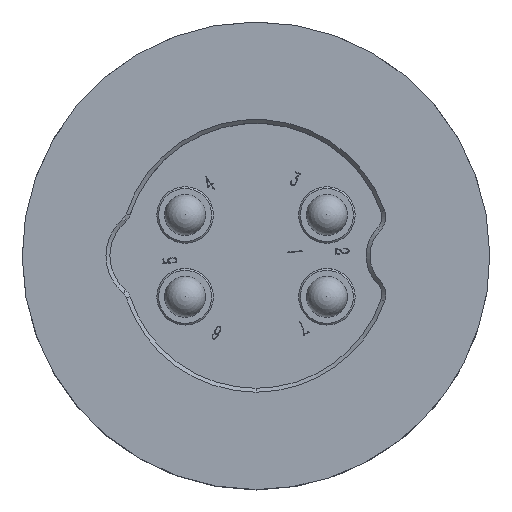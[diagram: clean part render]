
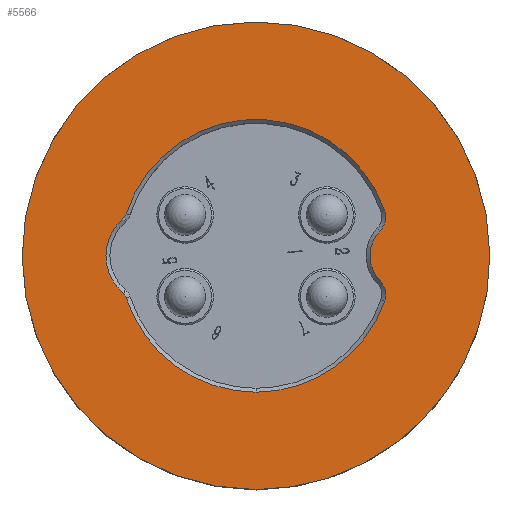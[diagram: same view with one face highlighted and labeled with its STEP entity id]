
A CAD part, top view. The second image highlights one B-rep face of the part: STEP entity #5566.
In plain terms, the highlighted planar face has unit normal (0, 0, 1).
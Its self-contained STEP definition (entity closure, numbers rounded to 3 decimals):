
#47 = DIRECTION ( 'NONE',  ( -1., 0., 0. ) ) ;
#152 = CARTESIAN_POINT ( 'NONE',  ( 0., 0., 0. ) ) ;
#515 = AXIS2_PLACEMENT_3D ( 'NONE', #9456, #1207, #4871 ) ;
#540 = EDGE_CURVE ( 'NONE', #8678, #10685, #4382, .T. ) ;
#756 = CARTESIAN_POINT ( 'NONE',  ( 0., -3.5, 0. ) ) ;
#1207 = DIRECTION ( 'NONE',  ( 0., 0., 1. ) ) ;
#1212 = CARTESIAN_POINT ( 'NONE',  ( 0., 0., 0. ) ) ;
#1215 = DIRECTION ( 'NONE',  ( 0., 0., 1. ) ) ;
#1306 = DIRECTION ( 'NONE',  ( 0.943, -0.332, 0. ) ) ;
#1320 = CARTESIAN_POINT ( 'NONE',  ( -2.6, 0., 0. ) ) ;
#1339 = AXIS2_PLACEMENT_3D ( 'NONE', #9462, #1215, #4879 ) ;
#1507 = EDGE_CURVE ( 'NONE', #4298, #8516, #7248, .T. ) ;
#1793 = ORIENTED_EDGE ( 'NONE', *, *, #2219, .T. ) ;
#1893 = AXIS2_PLACEMENT_3D ( 'NONE', #1320, #4993, #8657 ) ;
#1932 = ORIENTED_EDGE ( 'NONE', *, *, #11006, .T. ) ;
#2031 = CARTESIAN_POINT ( 'NONE',  ( -3.33, -1.079, 0. ) ) ;
#2101 = EDGE_CURVE ( 'NONE', #4407, #4084, #5161, .T. ) ;
#2219 = EDGE_CURVE ( 'NONE', #4084, #4665, #7648, .T. ) ;
#2424 = DIRECTION ( 'NONE',  ( 0.943, -0.332, 0. ) ) ;
#2466 = AXIS2_PLACEMENT_3D ( 'NONE', #11554, #3294, #6956 ) ;
#2517 = DIRECTION ( 'NONE',  ( 0., -1., 0. ) ) ;
#2592 = DIRECTION ( 'NONE',  ( 0.716, 0.698, 0. ) ) ;
#2992 = EDGE_LOOP ( 'NONE', ( #5444, #9931, #11263 ) ) ;
#3232 = VERTEX_POINT ( 'NONE', #7634 ) ;
#3294 = DIRECTION ( 'NONE',  ( 0., 0., -1. ) ) ;
#3421 = AXIS2_PLACEMENT_3D ( 'NONE', #4634, #8295, #47 ) ;
#3426 = PLANE ( 'NONE',  #9767 ) ;
#3532 = DIRECTION ( 'NONE',  ( 0., 0., 1. ) ) ;
#3622 = AXIS2_PLACEMENT_3D ( 'NONE', #11799, #3532, #7199 ) ;
#3653 = CIRCLE ( 'NONE', #10380, 0.5 ) ;
#3708 = CARTESIAN_POINT ( 'NONE',  ( 0., 0., 0. ) ) ;
#3765 = ORIENTED_EDGE ( 'NONE', *, *, #540, .T. ) ;
#3799 = ORIENTED_EDGE ( 'NONE', *, *, #1507, .T. ) ;
#3841 = DIRECTION ( 'NONE',  ( 0., 0., -1. ) ) ;
#4084 = VERTEX_POINT ( 'NONE', #7166 ) ;
#4183 = CARTESIAN_POINT ( 'NONE',  ( -3.419, -0.945, 0. ) ) ;
#4298 = VERTEX_POINT ( 'NONE', #2031 ) ;
#4348 = ORIENTED_EDGE ( 'NONE', *, *, #9005, .T. ) ;
#4382 = CIRCLE ( 'NONE', #7444, 3.5 ) ;
#4407 = VERTEX_POINT ( 'NONE', #10471 ) ;
#4442 = EDGE_CURVE ( 'NONE', #8516, #3232, #7078, .T. ) ;
#4526 = ORIENTED_EDGE ( 'NONE', *, *, #11235, .T. ) ;
#4616 = VERTEX_POINT ( 'NONE', #8228 ) ;
#4634 = CARTESIAN_POINT ( 'NONE',  ( 3.85, 0., 0. ) ) ;
#4665 = VERTEX_POINT ( 'NONE', #5587 ) ;
#4871 = DIRECTION ( 'NONE',  ( 0.951, 0.308, 0. ) ) ;
#4875 = DIRECTION ( 'NONE',  ( 0., 0., 1. ) ) ;
#4879 = DIRECTION ( 'NONE',  ( 0.655, -0.756, 0. ) ) ;
#4993 = DIRECTION ( 'NONE',  ( 0., 0., -1. ) ) ;
#4999 = CARTESIAN_POINT ( 'NONE',  ( 3.188, -0.646, 0. ) ) ;
#5017 = EDGE_CURVE ( 'NONE', #4616, #8506, #10330, .T. ) ;
#5131 = AXIS2_PLACEMENT_3D ( 'NONE', #1212, #4875, #8536 ) ;
#5161 = CIRCLE ( 'NONE', #11907, 3.5 ) ;
#5343 = AXIS2_PLACEMENT_3D ( 'NONE', #5869, #9549, #1306 ) ;
#5444 = ORIENTED_EDGE ( 'NONE', *, *, #9141, .T. ) ;
#5566 = ADVANCED_FACE ( 'NONE', ( #7988, #11687 ), #3426, .F. ) ;
#5587 = CARTESIAN_POINT ( 'NONE',  ( 3.188, 0.646, 0. ) ) ;
#5676 = EDGE_CURVE ( 'NONE', #4665, #9654, #8591, .T. ) ;
#5869 = CARTESIAN_POINT ( 'NONE',  ( 0., 0., 0. ) ) ;
#5938 = CIRCLE ( 'NONE', #7476, 6. ) ;
#6522 = CIRCLE ( 'NONE', #1339, 0.3 ) ;
#6956 = DIRECTION ( 'NONE',  ( 0.943, 0.332, 0. ) ) ;
#7005 = CARTESIAN_POINT ( 'NONE',  ( 0., 0., 0. ) ) ;
#7078 = CIRCLE ( 'NONE', #1893, 1.25 ) ;
#7100 = CARTESIAN_POINT ( 'NONE',  ( 4.25, 0.028, 0. ) ) ;
#7166 = CARTESIAN_POINT ( 'NONE',  ( 3.302, 1.161, 0. ) ) ;
#7181 = CARTESIAN_POINT ( 'NONE',  ( 2.83, -0.995, 0. ) ) ;
#7199 = DIRECTION ( 'NONE',  ( 1., 0.007, 0. ) ) ;
#7248 = CIRCLE ( 'NONE', #515, 0.3 ) ;
#7370 = DIRECTION ( 'NONE',  ( 0., 0., 1. ) ) ;
#7444 = AXIS2_PLACEMENT_3D ( 'NONE', #7005, #10697, #2424 ) ;
#7476 = AXIS2_PLACEMENT_3D ( 'NONE', #3708, #7370, #11059 ) ;
#7502 = DIRECTION ( 'NONE',  ( -0.951, 0.308, 0. ) ) ;
#7634 = CARTESIAN_POINT ( 'NONE',  ( -3.419, 0.945, 0. ) ) ;
#7648 = CIRCLE ( 'NONE', #2466, 0.5 ) ;
#7784 = ORIENTED_EDGE ( 'NONE', *, *, #2101, .T. ) ;
#7988 = FACE_OUTER_BOUND ( 'NONE', #2992, .T. ) ;
#8228 = CARTESIAN_POINT ( 'NONE',  ( 0., -6., 0. ) ) ;
#8295 = DIRECTION ( 'NONE',  ( 0., 0., 1. ) ) ;
#8506 = VERTEX_POINT ( 'NONE', #8634 ) ;
#8516 = VERTEX_POINT ( 'NONE', #4183 ) ;
#8536 = DIRECTION ( 'NONE',  ( -1., -0.007, 0. ) ) ;
#8591 = CIRCLE ( 'NONE', #3421, 0.925 ) ;
#8634 = CARTESIAN_POINT ( 'NONE',  ( 6., 0.04, 0. ) ) ;
#8657 = DIRECTION ( 'NONE',  ( -1., 0., 0. ) ) ;
#8678 = VERTEX_POINT ( 'NONE', #11838 ) ;
#8802 = CIRCLE ( 'NONE', #3622, 6. ) ;
#9005 = EDGE_CURVE ( 'NONE', #10685, #4298, #10539, .T. ) ;
#9141 = EDGE_CURVE ( 'NONE', #8506, #10467, #8802, .T. ) ;
#9456 = CARTESIAN_POINT ( 'NONE',  ( -3.615, -1.172, 0. ) ) ;
#9462 = CARTESIAN_POINT ( 'NONE',  ( -3.615, 1.172, 0. ) ) ;
#9549 = DIRECTION ( 'NONE',  ( 0., 0., -1. ) ) ;
#9654 = VERTEX_POINT ( 'NONE', #4999 ) ;
#9767 = AXIS2_PLACEMENT_3D ( 'NONE', #7100, #10792, #2517 ) ;
#9835 = ORIENTED_EDGE ( 'NONE', *, *, #5676, .T. ) ;
#9931 = ORIENTED_EDGE ( 'NONE', *, *, #10786, .T. ) ;
#10330 = CIRCLE ( 'NONE', #5131, 6. ) ;
#10380 = AXIS2_PLACEMENT_3D ( 'NONE', #7181, #10869, #2592 ) ;
#10454 = CARTESIAN_POINT ( 'NONE',  ( -6., -0.04, 0. ) ) ;
#10467 = VERTEX_POINT ( 'NONE', #10454 ) ;
#10471 = CARTESIAN_POINT ( 'NONE',  ( -3.33, 1.079, 0. ) ) ;
#10539 = CIRCLE ( 'NONE', #5343, 3.5 ) ;
#10685 = VERTEX_POINT ( 'NONE', #756 ) ;
#10697 = DIRECTION ( 'NONE',  ( 0., 0., -1. ) ) ;
#10786 = EDGE_CURVE ( 'NONE', #10467, #4616, #5938, .T. ) ;
#10792 = DIRECTION ( 'NONE',  ( 0., 0., -1. ) ) ;
#10869 = DIRECTION ( 'NONE',  ( 0., 0., -1. ) ) ;
#10921 = EDGE_LOOP ( 'NONE', ( #1793, #9835, #1932, #3765, #4348, #3799, #11144, #4526, #7784 ) ) ;
#11006 = EDGE_CURVE ( 'NONE', #9654, #8678, #3653, .T. ) ;
#11059 = DIRECTION ( 'NONE',  ( -1., -0.007, 0. ) ) ;
#11144 = ORIENTED_EDGE ( 'NONE', *, *, #4442, .T. ) ;
#11235 = EDGE_CURVE ( 'NONE', #3232, #4407, #6522, .T. ) ;
#11263 = ORIENTED_EDGE ( 'NONE', *, *, #5017, .T. ) ;
#11554 = CARTESIAN_POINT ( 'NONE',  ( 2.83, 0.995, 0. ) ) ;
#11687 = FACE_BOUND ( 'NONE', #10921, .T. ) ;
#11799 = CARTESIAN_POINT ( 'NONE',  ( 0., 0., 0. ) ) ;
#11838 = CARTESIAN_POINT ( 'NONE',  ( 3.302, -1.161, 0. ) ) ;
#11907 = AXIS2_PLACEMENT_3D ( 'NONE', #152, #3841, #7502 ) ;
